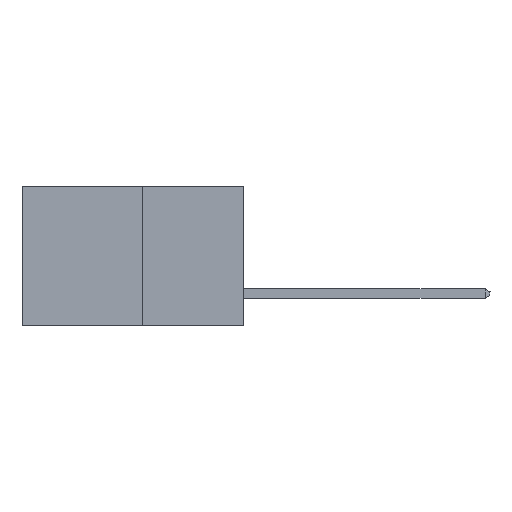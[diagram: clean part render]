
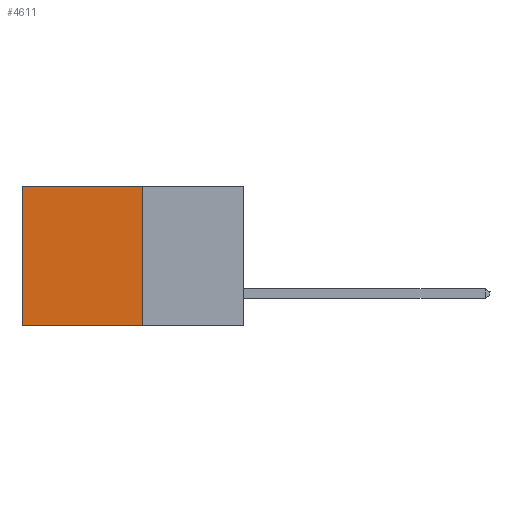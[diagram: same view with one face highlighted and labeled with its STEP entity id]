
A CAD part, left-side view. The second image highlights one B-rep face of the part: STEP entity #4611.
In plain terms, the highlighted planar face has unit normal (-1, 0, 0).
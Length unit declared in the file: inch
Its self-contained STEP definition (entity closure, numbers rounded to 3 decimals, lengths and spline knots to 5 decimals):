
#1679 = DIRECTION ( 'NONE',  ( 0., 1., 0. ) ) ;
#2897 = CARTESIAN_POINT ( 'NONE',  ( 0.277, 0.59, -0.37 ) ) ;
#3425 = EDGE_CURVE ( 'NONE', #16043, #11418, #9736, .T. ) ;
#3469 = LINE ( 'NONE', #16550, #6937 ) ;
#3603 = DIRECTION ( 'NONE',  ( 0., 1., 0. ) ) ;
#4611 = ADVANCED_FACE ( 'NONE', ( #6837 ), #6203, .F. ) ;
#5128 = ORIENTED_EDGE ( 'NONE', *, *, #15216, .F. ) ;
#5982 = CARTESIAN_POINT ( 'NONE',  ( 0.277, 0.27, -0.37 ) ) ;
#6021 = DIRECTION ( 'NONE',  ( 0., 0., -1. ) ) ;
#6203 = PLANE ( 'NONE',  #15731 ) ;
#6837 = FACE_OUTER_BOUND ( 'NONE', #16085, .T. ) ;
#6937 = VECTOR ( 'NONE', #6021, 39.37008 ) ;
#6945 = CARTESIAN_POINT ( 'NONE',  ( 0.277, 0.27, -0.37 ) ) ;
#7485 = ORIENTED_EDGE ( 'NONE', *, *, #11698, .F. ) ;
#7558 = DIRECTION ( 'NONE',  ( 0., 0., -1. ) ) ;
#8243 = CARTESIAN_POINT ( 'NONE',  ( 0.277, 0.27, 0. ) ) ;
#8377 = ORIENTED_EDGE ( 'NONE', *, *, #10221, .T. ) ;
#9418 = DIRECTION ( 'NONE',  ( 0., 0., -1. ) ) ;
#9736 = LINE ( 'NONE', #15328, #16318 ) ;
#10008 = LINE ( 'NONE', #6945, #13130 ) ;
#10221 = EDGE_CURVE ( 'NONE', #11418, #11324, #11717, .T. ) ;
#10455 = VERTEX_POINT ( 'NONE', #5982 ) ;
#11314 = VECTOR ( 'NONE', #9418, 39.37008 ) ;
#11324 = VERTEX_POINT ( 'NONE', #12124 ) ;
#11418 = VERTEX_POINT ( 'NONE', #15654 ) ;
#11592 = ORIENTED_EDGE ( 'NONE', *, *, #3425, .T. ) ;
#11698 = EDGE_CURVE ( 'NONE', #10455, #11324, #10008, .T. ) ;
#11717 = LINE ( 'NONE', #2897, #11314 ) ;
#12124 = CARTESIAN_POINT ( 'NONE',  ( 0.277, 0.59, -0.37 ) ) ;
#13130 = VECTOR ( 'NONE', #1679, 39.37008 ) ;
#14148 = CARTESIAN_POINT ( 'NONE',  ( 0.277, 0.27, -0.37 ) ) ;
#15216 = EDGE_CURVE ( 'NONE', #16043, #10455, #3469, .T. ) ;
#15328 = CARTESIAN_POINT ( 'NONE',  ( 0.277, 0.27, 0. ) ) ;
#15461 = DIRECTION ( 'NONE',  ( 1., 0., 0. ) ) ;
#15654 = CARTESIAN_POINT ( 'NONE',  ( 0.277, 0.59, 0. ) ) ;
#15731 = AXIS2_PLACEMENT_3D ( 'NONE', #14148, #15461, #7558 ) ;
#16043 = VERTEX_POINT ( 'NONE', #8243 ) ;
#16085 = EDGE_LOOP ( 'NONE', ( #8377, #7485, #5128, #11592 ) ) ;
#16318 = VECTOR ( 'NONE', #3603, 39.37008 ) ;
#16550 = CARTESIAN_POINT ( 'NONE',  ( 0.277, 0.27, -0.37 ) ) ;
